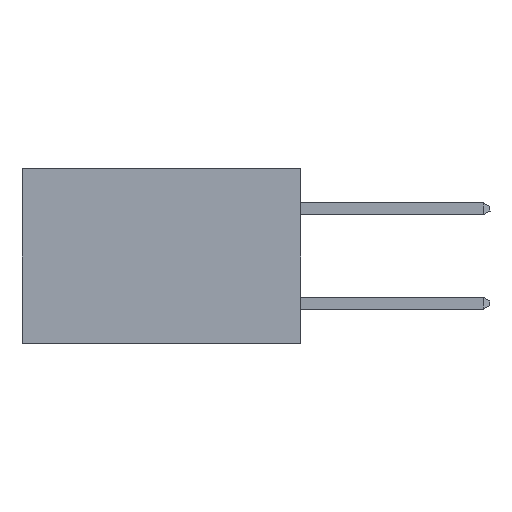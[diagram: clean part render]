
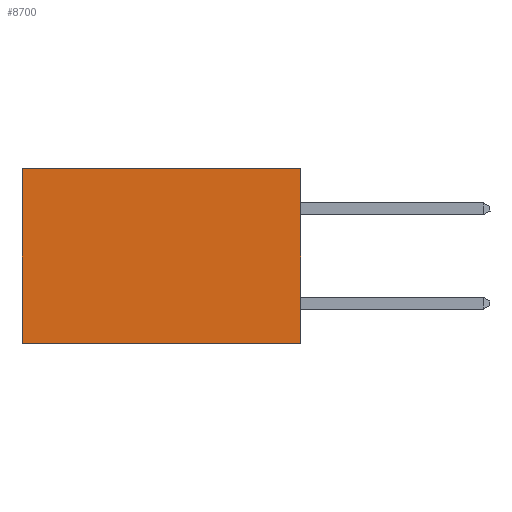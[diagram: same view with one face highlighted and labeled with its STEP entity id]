
A CAD part, left-side view. The second image highlights one B-rep face of the part: STEP entity #8700.
In plain terms, the highlighted planar face has unit normal (-1, 0, 0).
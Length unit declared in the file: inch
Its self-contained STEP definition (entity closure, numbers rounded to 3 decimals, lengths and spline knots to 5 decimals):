
#1943 = CARTESIAN_POINT ( 'NONE',  ( 0.277, 0., -0.37 ) ) ;
#1996 = AXIS2_PLACEMENT_3D ( 'NONE', #8449, #8118, #8098 ) ;
#2069 = ORIENTED_EDGE ( 'NONE', *, *, #24254, .T. ) ;
#2121 = ORIENTED_EDGE ( 'NONE', *, *, #9771, .F. ) ;
#2830 = VERTEX_POINT ( 'NONE', #18791 ) ;
#2900 = EDGE_LOOP ( 'NONE', ( #3937, #2121, #8384, #2069 ) ) ;
#3785 = FACE_OUTER_BOUND ( 'NONE', #2900, .T. ) ;
#3937 = ORIENTED_EDGE ( 'NONE', *, *, #17165, .T. ) ;
#4180 = VECTOR ( 'NONE', #9448, 39.37008 ) ;
#5937 = LINE ( 'NONE', #13622, #11447 ) ;
#6864 = EDGE_CURVE ( 'NONE', #2830, #9176, #22566, .T. ) ;
#6976 = VECTOR ( 'NONE', #25509, 39.37008 ) ;
#8098 = DIRECTION ( 'NONE',  ( 0., 0., -1. ) ) ;
#8118 = DIRECTION ( 'NONE',  ( 1., 0., 0. ) ) ;
#8384 = ORIENTED_EDGE ( 'NONE', *, *, #6864, .F. ) ;
#8449 = CARTESIAN_POINT ( 'NONE',  ( 0.277, 0., -0.37 ) ) ;
#8597 = PLANE ( 'NONE',  #1996 ) ;
#8700 = ADVANCED_FACE ( 'NONE', ( #3785 ), #8597, .F. ) ;
#9176 = VERTEX_POINT ( 'NONE', #1943 ) ;
#9448 = DIRECTION ( 'NONE',  ( 0., 0., -1. ) ) ;
#9771 = EDGE_CURVE ( 'NONE', #9176, #25536, #5937, .T. ) ;
#11447 = VECTOR ( 'NONE', #13531, 39.37008 ) ;
#11543 = CARTESIAN_POINT ( 'NONE',  ( 0.277, 0., 0. ) ) ;
#13357 = VERTEX_POINT ( 'NONE', #19682 ) ;
#13387 = DIRECTION ( 'NONE',  ( 0., 0., -1. ) ) ;
#13531 = DIRECTION ( 'NONE',  ( 0., 1., 0. ) ) ;
#13622 = CARTESIAN_POINT ( 'NONE',  ( 0.277, 0., -0.37 ) ) ;
#13680 = CARTESIAN_POINT ( 'NONE',  ( 0.277, 0., -0.37 ) ) ;
#15138 = LINE ( 'NONE', #23544, #4180 ) ;
#17165 = EDGE_CURVE ( 'NONE', #13357, #25536, #15138, .T. ) ;
#18791 = CARTESIAN_POINT ( 'NONE',  ( 0.277, 0., 0. ) ) ;
#19682 = CARTESIAN_POINT ( 'NONE',  ( 0.277, 0.59, 0. ) ) ;
#21948 = VECTOR ( 'NONE', #13387, 39.37008 ) ;
#22566 = LINE ( 'NONE', #13680, #21948 ) ;
#23544 = CARTESIAN_POINT ( 'NONE',  ( 0.277, 0.59, -0.37 ) ) ;
#24254 = EDGE_CURVE ( 'NONE', #2830, #13357, #24373, .T. ) ;
#24373 = LINE ( 'NONE', #11543, #6976 ) ;
#25367 = CARTESIAN_POINT ( 'NONE',  ( 0.277, 0.59, -0.37 ) ) ;
#25509 = DIRECTION ( 'NONE',  ( 0., 1., 0. ) ) ;
#25536 = VERTEX_POINT ( 'NONE', #25367 ) ;
